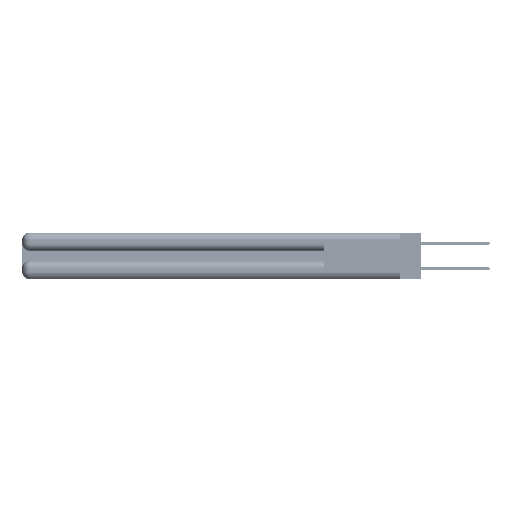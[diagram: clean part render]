
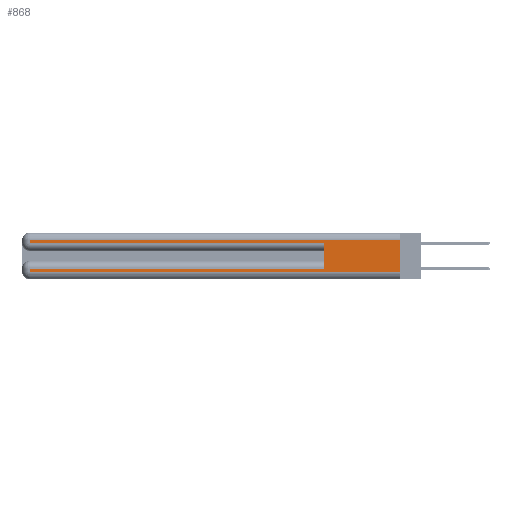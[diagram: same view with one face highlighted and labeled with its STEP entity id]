
A CAD part, left-side view. The second image highlights one B-rep face of the part: STEP entity #868.
In plain terms, the highlighted planar face has unit normal (-1, 0, 0).
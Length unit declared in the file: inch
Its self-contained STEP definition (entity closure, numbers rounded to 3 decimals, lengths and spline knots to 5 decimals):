
#383 = VERTEX_POINT ( 'NONE', #9265 ) ;
#405 = EDGE_CURVE ( 'NONE', #383, #11436, #42175, .T. ) ;
#416 = ORIENTED_EDGE ( 'NONE', *, *, #43714, .F. ) ;
#868 = ADVANCED_FACE ( 'NONE', ( #42847 ), #55209, .F. ) ;
#881 = EDGE_CURVE ( 'NONE', #34337, #6868, #25949, .T. ) ;
#2356 = VECTOR ( 'NONE', #30573, 39.37008 ) ;
#3580 = LINE ( 'NONE', #31013, #17049 ) ;
#4291 = DIRECTION ( 'NONE',  ( 0., 0., -1. ) ) ;
#4769 = LINE ( 'NONE', #14487, #26377 ) ;
#4870 = CARTESIAN_POINT ( 'NONE',  ( 0., 2.94, 0.31 ) ) ;
#6164 = CARTESIAN_POINT ( 'NONE',  ( 0., 0.6, 0.285 ) ) ;
#6868 = VERTEX_POINT ( 'NONE', #53918 ) ;
#7514 = DIRECTION ( 'NONE',  ( 0., 0., -1. ) ) ;
#7888 = DIRECTION ( 'NONE',  ( 1., 0., 0. ) ) ;
#9265 = CARTESIAN_POINT ( 'NONE',  ( 0., 0.6, 0.085 ) ) ;
#11436 = VERTEX_POINT ( 'NONE', #37423 ) ;
#12250 = LINE ( 'NONE', #27109, #38571 ) ;
#12256 = LINE ( 'NONE', #14889, #53427 ) ;
#12555 = CARTESIAN_POINT ( 'NONE',  ( 0., 2.94, 0.06 ) ) ;
#12740 = ORIENTED_EDGE ( 'NONE', *, *, #49874, .T. ) ;
#12941 = ORIENTED_EDGE ( 'NONE', *, *, #32803, .T. ) ;
#13302 = DIRECTION ( 'NONE',  ( 0., 0., -1. ) ) ;
#14487 = CARTESIAN_POINT ( 'NONE',  ( 0., 0., 0.285 ) ) ;
#14889 = CARTESIAN_POINT ( 'NONE',  ( 0., 0., 0.37 ) ) ;
#16748 = CARTESIAN_POINT ( 'NONE',  ( 0., 2.94, 0.37 ) ) ;
#17049 = VECTOR ( 'NONE', #27416, 39.37008 ) ;
#20871 = EDGE_CURVE ( 'NONE', #11436, #22290, #53518, .T. ) ;
#21218 = VECTOR ( 'NONE', #23644, 39.37008 ) ;
#22290 = VERTEX_POINT ( 'NONE', #12555 ) ;
#23644 = DIRECTION ( 'NONE',  ( 0., 0., 1. ) ) ;
#24414 = ORIENTED_EDGE ( 'NONE', *, *, #881, .T. ) ;
#24579 = ORIENTED_EDGE ( 'NONE', *, *, #405, .T. ) ;
#25949 = LINE ( 'NONE', #16748, #52945 ) ;
#26377 = VECTOR ( 'NONE', #27489, 39.37008 ) ;
#26981 = CARTESIAN_POINT ( 'NONE',  ( 0., 0., 0.085 ) ) ;
#27109 = CARTESIAN_POINT ( 'NONE',  ( 0., 0., 0.06 ) ) ;
#27273 = AXIS2_PLACEMENT_3D ( 'NONE', #33736, #7888, #7514 ) ;
#27416 = DIRECTION ( 'NONE',  ( 0., 1., 0. ) ) ;
#27489 = DIRECTION ( 'NONE',  ( 0., -1., 0. ) ) ;
#30486 = EDGE_CURVE ( 'NONE', #383, #41276, #32716, .T. ) ;
#30518 = ORIENTED_EDGE ( 'NONE', *, *, #33964, .T. ) ;
#30573 = DIRECTION ( 'NONE',  ( 0., 1., 0. ) ) ;
#31013 = CARTESIAN_POINT ( 'NONE',  ( 0., 0., 0.31 ) ) ;
#32716 = LINE ( 'NONE', #49480, #21218 ) ;
#32803 = EDGE_CURVE ( 'NONE', #35442, #34337, #3580, .T. ) ;
#33416 = ORIENTED_EDGE ( 'NONE', *, *, #20871, .T. ) ;
#33736 = CARTESIAN_POINT ( 'NONE',  ( 0., 0., 0.37 ) ) ;
#33964 = EDGE_CURVE ( 'NONE', #6868, #41276, #4769, .T. ) ;
#34337 = VERTEX_POINT ( 'NONE', #4870 ) ;
#34793 = EDGE_LOOP ( 'NONE', ( #416, #12941, #24414, #30518, #41719, #24579, #33416, #12740 ) ) ;
#35442 = VERTEX_POINT ( 'NONE', #51323 ) ;
#35832 = DIRECTION ( 'NONE',  ( 0., -1., 0. ) ) ;
#36354 = VERTEX_POINT ( 'NONE', #49171 ) ;
#37423 = CARTESIAN_POINT ( 'NONE',  ( 0., 2.94, 0.085 ) ) ;
#38571 = VECTOR ( 'NONE', #35832, 39.37008 ) ;
#39352 = CARTESIAN_POINT ( 'NONE',  ( 0., 2.94, 0.37 ) ) ;
#41276 = VERTEX_POINT ( 'NONE', #6164 ) ;
#41719 = ORIENTED_EDGE ( 'NONE', *, *, #30486, .F. ) ;
#42175 = LINE ( 'NONE', #26981, #2356 ) ;
#42847 = FACE_OUTER_BOUND ( 'NONE', #34793, .T. ) ;
#43714 = EDGE_CURVE ( 'NONE', #35442, #36354, #12256, .T. ) ;
#45434 = VECTOR ( 'NONE', #13302, 39.37008 ) ;
#49171 = CARTESIAN_POINT ( 'NONE',  ( 0., 0., 0.06 ) ) ;
#49398 = DIRECTION ( 'NONE',  ( 0., 0., -1. ) ) ;
#49480 = CARTESIAN_POINT ( 'NONE',  ( 0., 0.6, 0.145 ) ) ;
#49874 = EDGE_CURVE ( 'NONE', #22290, #36354, #12250, .T. ) ;
#51323 = CARTESIAN_POINT ( 'NONE',  ( 0., 0., 0.31 ) ) ;
#52945 = VECTOR ( 'NONE', #4291, 39.37008 ) ;
#53427 = VECTOR ( 'NONE', #49398, 39.37008 ) ;
#53518 = LINE ( 'NONE', #39352, #45434 ) ;
#53918 = CARTESIAN_POINT ( 'NONE',  ( 0., 2.94, 0.285 ) ) ;
#55209 = PLANE ( 'NONE',  #27273 ) ;
